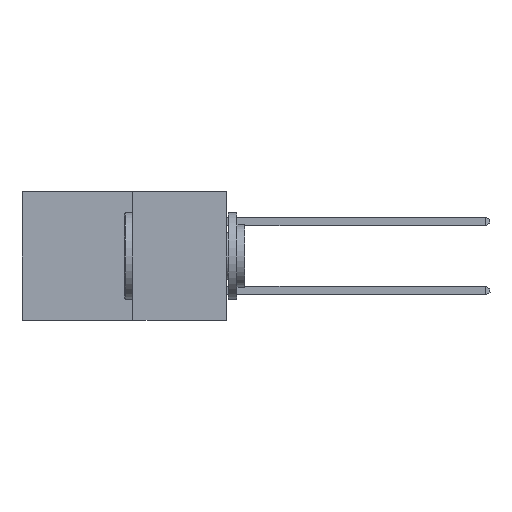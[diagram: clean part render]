
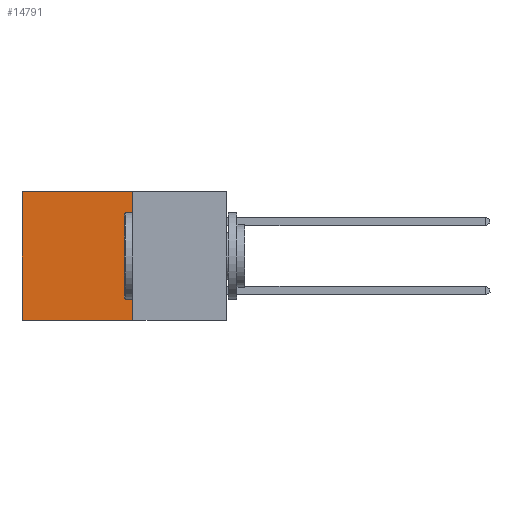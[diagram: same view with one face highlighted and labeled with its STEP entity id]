
A CAD part, left-side view. The second image highlights one B-rep face of the part: STEP entity #14791.
In plain terms, the highlighted planar face has unit normal (-1, 0, 0).
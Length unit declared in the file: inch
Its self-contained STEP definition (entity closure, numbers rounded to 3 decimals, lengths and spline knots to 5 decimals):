
#1023 = EDGE_CURVE ( 'NONE', #12378, #12611, #26706, .T. ) ;
#1036 = AXIS2_PLACEMENT_3D ( 'NONE', #13231, #13440, #29979 ) ;
#2917 = EDGE_CURVE ( 'NONE', #27483, #12378, #5582, .T. ) ;
#4191 = CARTESIAN_POINT ( 'NONE',  ( 0.277, 0.27, 0. ) ) ;
#5038 = CARTESIAN_POINT ( 'NONE',  ( 0.277, 0.59, 0. ) ) ;
#5582 = LINE ( 'NONE', #18601, #24102 ) ;
#7938 = CARTESIAN_POINT ( 'NONE',  ( 0.277, 0.27, -0.37 ) ) ;
#8622 = EDGE_CURVE ( 'NONE', #27483, #8886, #16995, .T. ) ;
#8775 = CARTESIAN_POINT ( 'NONE',  ( 0.277, 0.59, -0.37 ) ) ;
#8886 = VERTEX_POINT ( 'NONE', #5038 ) ;
#9801 = ORIENTED_EDGE ( 'NONE', *, *, #24128, .T. ) ;
#12378 = VERTEX_POINT ( 'NONE', #15401 ) ;
#12611 = VERTEX_POINT ( 'NONE', #8775 ) ;
#13205 = DIRECTION ( 'NONE',  ( 0., 0., -1. ) ) ;
#13231 = CARTESIAN_POINT ( 'NONE',  ( 0.277, 0.27, -0.37 ) ) ;
#13440 = DIRECTION ( 'NONE',  ( 1., 0., 0. ) ) ;
#13834 = ORIENTED_EDGE ( 'NONE', *, *, #1023, .F. ) ;
#14029 = EDGE_LOOP ( 'NONE', ( #9801, #13834, #24242, #27942 ) ) ;
#14791 = ADVANCED_FACE ( 'NONE', ( #28574 ), #27638, .F. ) ;
#15401 = CARTESIAN_POINT ( 'NONE',  ( 0.277, 0.27, -0.37 ) ) ;
#15489 = VECTOR ( 'NONE', #23383, 39.37008 ) ;
#15952 = DIRECTION ( 'NONE',  ( 0., 1., 0. ) ) ;
#16035 = DIRECTION ( 'NONE',  ( 0., 0., -1. ) ) ;
#16995 = LINE ( 'NONE', #23274, #15489 ) ;
#18601 = CARTESIAN_POINT ( 'NONE',  ( 0.277, 0.27, -0.37 ) ) ;
#21992 = VECTOR ( 'NONE', #15952, 39.37008 ) ;
#22450 = VECTOR ( 'NONE', #13205, 39.37008 ) ;
#23274 = CARTESIAN_POINT ( 'NONE',  ( 0.277, 0.27, 0. ) ) ;
#23383 = DIRECTION ( 'NONE',  ( 0., 1., 0. ) ) ;
#24102 = VECTOR ( 'NONE', #16035, 39.37008 ) ;
#24128 = EDGE_CURVE ( 'NONE', #8886, #12611, #27920, .T. ) ;
#24242 = ORIENTED_EDGE ( 'NONE', *, *, #2917, .F. ) ;
#25081 = CARTESIAN_POINT ( 'NONE',  ( 0.277, 0.59, -0.37 ) ) ;
#26706 = LINE ( 'NONE', #7938, #21992 ) ;
#27483 = VERTEX_POINT ( 'NONE', #4191 ) ;
#27638 = PLANE ( 'NONE',  #1036 ) ;
#27920 = LINE ( 'NONE', #25081, #22450 ) ;
#27942 = ORIENTED_EDGE ( 'NONE', *, *, #8622, .T. ) ;
#28574 = FACE_OUTER_BOUND ( 'NONE', #14029, .T. ) ;
#29979 = DIRECTION ( 'NONE',  ( 0., 0., -1. ) ) ;
